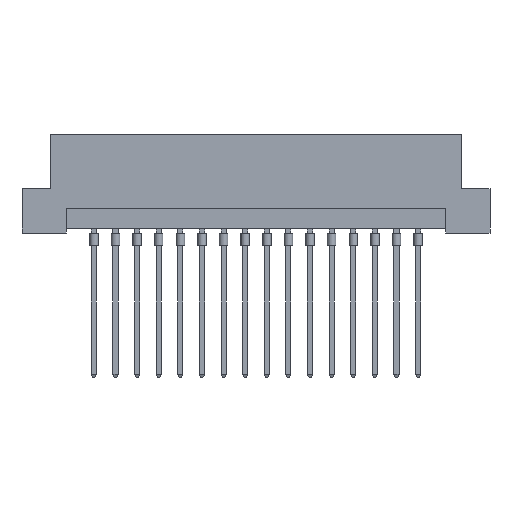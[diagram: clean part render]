
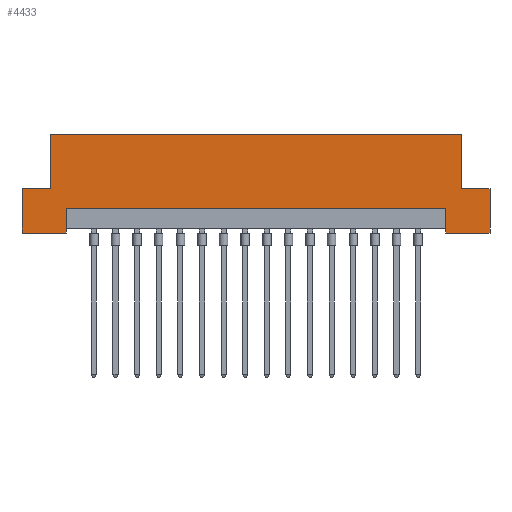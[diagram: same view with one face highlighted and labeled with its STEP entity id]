
A CAD part, front view. The second image highlights one B-rep face of the part: STEP entity #4433.
In plain terms, the highlighted planar face has unit normal (0, -1, 0).
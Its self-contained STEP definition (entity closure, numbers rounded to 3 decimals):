
#89 = CARTESIAN_POINT ( 'NONE',  ( -27.5, 0., 0. ) ) ;
#486 = LINE ( 'NONE', #7496, #3099 ) ;
#747 = LINE ( 'NONE', #4659, #6191 ) ;
#864 = ORIENTED_EDGE ( 'NONE', *, *, #4730, .F. ) ;
#895 = CARTESIAN_POINT ( 'NONE',  ( -27.5, 0., 0. ) ) ;
#1244 = LINE ( 'NONE', #3571, #6406 ) ;
#1327 = DIRECTION ( 'NONE',  ( 0., 0., 1. ) ) ;
#1330 = CARTESIAN_POINT ( 'NONE',  ( 22.3, 0., 0.5 ) ) ;
#1344 = VECTOR ( 'NONE', #9446, 1000. ) ;
#1387 = DIRECTION ( 'NONE',  ( 0., 0., 1. ) ) ;
#1574 = EDGE_CURVE ( 'NONE', #5798, #8676, #8823, .T. ) ;
#1774 = DIRECTION ( 'NONE',  ( 0., 0., 1. ) ) ;
#1871 = EDGE_CURVE ( 'NONE', #4716, #5422, #486, .T. ) ;
#1919 = VERTEX_POINT ( 'NONE', #8368 ) ;
#1981 = DIRECTION ( 'NONE',  ( 0., 1., 0. ) ) ;
#2079 = CARTESIAN_POINT ( 'NONE',  ( -27.5, 0., 11.6 ) ) ;
#2256 = EDGE_CURVE ( 'NONE', #4691, #9955, #7278, .T. ) ;
#2342 = VECTOR ( 'NONE', #7590, 1000. ) ;
#2359 = EDGE_CURVE ( 'NONE', #6622, #5422, #4429, .T. ) ;
#2441 = CARTESIAN_POINT ( 'NONE',  ( 27.5, 0., 0. ) ) ;
#2618 = ORIENTED_EDGE ( 'NONE', *, *, #3658, .F. ) ;
#2643 = VECTOR ( 'NONE', #1387, 1000. ) ;
#2667 = DIRECTION ( 'NONE',  ( 1., 0., 0. ) ) ;
#2673 = CARTESIAN_POINT ( 'NONE',  ( -24.2, 0., 5.2 ) ) ;
#2807 = FACE_OUTER_BOUND ( 'NONE', #8427, .T. ) ;
#2825 = DIRECTION ( 'NONE',  ( 0., 0., -1. ) ) ;
#3099 = VECTOR ( 'NONE', #4492, 1000. ) ;
#3369 = CARTESIAN_POINT ( 'NONE',  ( 27.5, 0., 5.2 ) ) ;
#3421 = DIRECTION ( 'NONE',  ( 0., 0., 1. ) ) ;
#3477 = CARTESIAN_POINT ( 'NONE',  ( -22.3, 0., 2.9 ) ) ;
#3571 = CARTESIAN_POINT ( 'NONE',  ( -22.3, 0., 0.5 ) ) ;
#3589 = VERTEX_POINT ( 'NONE', #895 ) ;
#3658 = EDGE_CURVE ( 'NONE', #6622, #8494, #8723, .T. ) ;
#3717 = CARTESIAN_POINT ( 'NONE',  ( -27.5, 0., 0. ) ) ;
#4171 = CARTESIAN_POINT ( 'NONE',  ( 22.3, 0., 2.9 ) ) ;
#4424 = DIRECTION ( 'NONE',  ( 0., 0., -1. ) ) ;
#4429 = LINE ( 'NONE', #7435, #2643 ) ;
#4433 = ADVANCED_FACE ( 'NONE', ( #2807 ), #6615, .F. ) ;
#4492 = DIRECTION ( 'NONE',  ( 1., 0., 0. ) ) ;
#4504 = ORIENTED_EDGE ( 'NONE', *, *, #2256, .F. ) ;
#4586 = VECTOR ( 'NONE', #3421, 1000. ) ;
#4659 = CARTESIAN_POINT ( 'NONE',  ( 22.3, 0., 2.9 ) ) ;
#4691 = VERTEX_POINT ( 'NONE', #7888 ) ;
#4716 = VERTEX_POINT ( 'NONE', #6308 ) ;
#4730 = EDGE_CURVE ( 'NONE', #3589, #4691, #9426, .T. ) ;
#4743 = EDGE_CURVE ( 'NONE', #8494, #5798, #7115, .T. ) ;
#4921 = CARTESIAN_POINT ( 'NONE',  ( -27.5, 0., 0. ) ) ;
#5005 = CARTESIAN_POINT ( 'NONE',  ( 24.2, 0., 11.6 ) ) ;
#5422 = VERTEX_POINT ( 'NONE', #5005 ) ;
#5537 = DIRECTION ( 'NONE',  ( 0., 0., -1. ) ) ;
#5556 = CARTESIAN_POINT ( 'NONE',  ( -24.2, 0., 5.2 ) ) ;
#5726 = CARTESIAN_POINT ( 'NONE',  ( 24.2, 0., 5.2 ) ) ;
#5732 = ORIENTED_EDGE ( 'NONE', *, *, #1871, .F. ) ;
#5798 = VERTEX_POINT ( 'NONE', #6045 ) ;
#5977 = VECTOR ( 'NONE', #1774, 1000. ) ;
#6045 = CARTESIAN_POINT ( 'NONE',  ( 27.5, 0., 0. ) ) ;
#6157 = VECTOR ( 'NONE', #2667, 1000. ) ;
#6158 = CARTESIAN_POINT ( 'NONE',  ( 27.5, 0., 5.2 ) ) ;
#6191 = VECTOR ( 'NONE', #9361, 1000. ) ;
#6308 = CARTESIAN_POINT ( 'NONE',  ( -24.2, 0., 11.6 ) ) ;
#6406 = VECTOR ( 'NONE', #2825, 1000. ) ;
#6479 = DIRECTION ( 'NONE',  ( -1., 0., 0. ) ) ;
#6615 = PLANE ( 'NONE',  #9100 ) ;
#6620 = ORIENTED_EDGE ( 'NONE', *, *, #8464, .F. ) ;
#6622 = VERTEX_POINT ( 'NONE', #5726 ) ;
#7115 = LINE ( 'NONE', #2441, #7439 ) ;
#7278 = LINE ( 'NONE', #9599, #1344 ) ;
#7370 = ORIENTED_EDGE ( 'NONE', *, *, #8075, .F. ) ;
#7398 = ORIENTED_EDGE ( 'NONE', *, *, #1574, .F. ) ;
#7435 = CARTESIAN_POINT ( 'NONE',  ( 24.2, 0., 5.2 ) ) ;
#7439 = VECTOR ( 'NONE', #5537, 1000. ) ;
#7443 = ORIENTED_EDGE ( 'NONE', *, *, #9032, .T. ) ;
#7496 = CARTESIAN_POINT ( 'NONE',  ( -27.5, 0., 11.6 ) ) ;
#7560 = ORIENTED_EDGE ( 'NONE', *, *, #4743, .F. ) ;
#7590 = DIRECTION ( 'NONE',  ( -1., 0., 0. ) ) ;
#7888 = CARTESIAN_POINT ( 'NONE',  ( -27.5, 0., 5.2 ) ) ;
#7929 = ORIENTED_EDGE ( 'NONE', *, *, #2359, .T. ) ;
#8075 = EDGE_CURVE ( 'NONE', #8886, #9743, #747, .T. ) ;
#8161 = LINE ( 'NONE', #2673, #4586 ) ;
#8178 = VECTOR ( 'NONE', #6479, 1000. ) ;
#8271 = EDGE_CURVE ( 'NONE', #9955, #4716, #8161, .T. ) ;
#8368 = CARTESIAN_POINT ( 'NONE',  ( -22.3, 0., 0. ) ) ;
#8380 = ORIENTED_EDGE ( 'NONE', *, *, #8431, .F. ) ;
#8427 = EDGE_LOOP ( 'NONE', ( #7370, #7443, #7398, #7560, #2618, #7929, #5732, #9803, #4504, #864, #6620, #8380 ) ) ;
#8431 = EDGE_CURVE ( 'NONE', #9743, #1919, #1244, .T. ) ;
#8464 = EDGE_CURVE ( 'NONE', #1919, #3589, #9906, .T. ) ;
#8494 = VERTEX_POINT ( 'NONE', #6158 ) ;
#8676 = VERTEX_POINT ( 'NONE', #9392 ) ;
#8723 = LINE ( 'NONE', #3369, #6157 ) ;
#8816 = VECTOR ( 'NONE', #4424, 1000. ) ;
#8823 = LINE ( 'NONE', #89, #8178 ) ;
#8886 = VERTEX_POINT ( 'NONE', #4171 ) ;
#9032 = EDGE_CURVE ( 'NONE', #8886, #8676, #9851, .T. ) ;
#9100 = AXIS2_PLACEMENT_3D ( 'NONE', #2079, #1981, #1327 ) ;
#9361 = DIRECTION ( 'NONE',  ( -1., 0., 0. ) ) ;
#9392 = CARTESIAN_POINT ( 'NONE',  ( 22.3, 0., 0. ) ) ;
#9426 = LINE ( 'NONE', #4921, #5977 ) ;
#9446 = DIRECTION ( 'NONE',  ( 1., 0., 0. ) ) ;
#9599 = CARTESIAN_POINT ( 'NONE',  ( -27.5, 0., 5.2 ) ) ;
#9743 = VERTEX_POINT ( 'NONE', #3477 ) ;
#9803 = ORIENTED_EDGE ( 'NONE', *, *, #8271, .F. ) ;
#9851 = LINE ( 'NONE', #1330, #8816 ) ;
#9906 = LINE ( 'NONE', #3717, #2342 ) ;
#9955 = VERTEX_POINT ( 'NONE', #5556 ) ;
